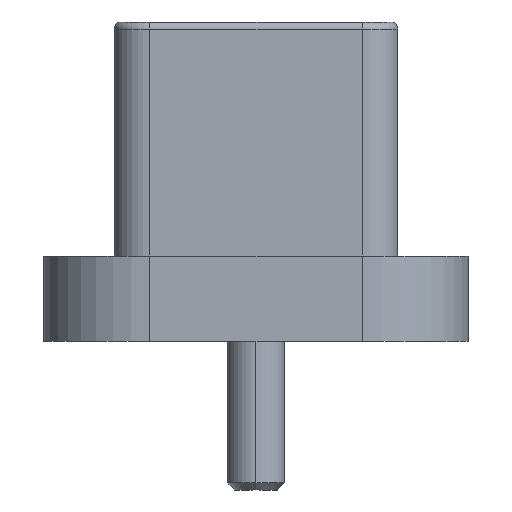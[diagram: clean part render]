
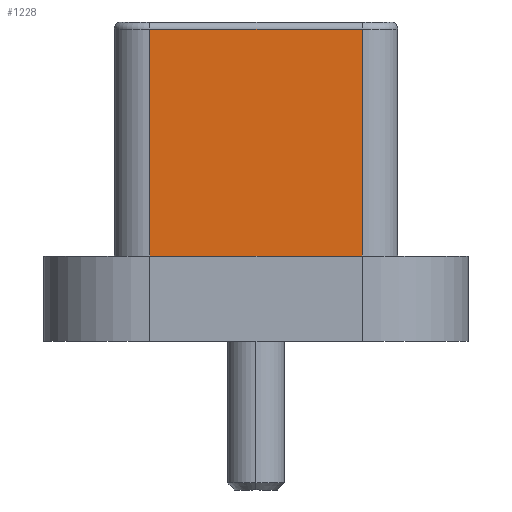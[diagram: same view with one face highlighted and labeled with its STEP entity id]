
A CAD part, left-side view. The second image highlights one B-rep face of the part: STEP entity #1228.
In plain terms, the highlighted planar face has unit normal (-1, 0, 0).
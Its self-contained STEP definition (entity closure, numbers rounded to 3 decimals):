
#111 = VERTEX_POINT ( 'NONE', #2740 ) ;
#316 = ORIENTED_EDGE ( 'NONE', *, *, #3835, .T. ) ;
#474 = CARTESIAN_POINT ( 'NONE',  ( -8.45, 1.5, -3.3 ) ) ;
#650 = LINE ( 'NONE', #2768, #5397 ) ;
#931 = VERTEX_POINT ( 'NONE', #3475 ) ;
#1100 = DIRECTION ( 'NONE',  ( 1., 0., 0. ) ) ;
#1228 = ADVANCED_FACE ( 'NONE', ( #1626 ), #3714, .F. ) ;
#1626 = FACE_OUTER_BOUND ( 'NONE', #5519, .T. ) ;
#1739 = VECTOR ( 'NONE', #6826, 1000. ) ;
#2544 = LINE ( 'NONE', #4677, #6033 ) ;
#2601 = DIRECTION ( 'NONE',  ( 0., -1., 0. ) ) ;
#2622 = LINE ( 'NONE', #4744, #1739 ) ;
#2649 = ORIENTED_EDGE ( 'NONE', *, *, #3925, .T. ) ;
#2740 = CARTESIAN_POINT ( 'NONE',  ( -8.45, 1.5, -3.3 ) ) ;
#2768 = CARTESIAN_POINT ( 'NONE',  ( -8.45, -1.5, -3.3 ) ) ;
#3069 = EDGE_CURVE ( 'NONE', #6422, #4673, #2622, .T. ) ;
#3185 = DIRECTION ( 'NONE',  ( 0., 1., 0. ) ) ;
#3358 = EDGE_CURVE ( 'NONE', #4673, #111, #2544, .T. ) ;
#3475 = CARTESIAN_POINT ( 'NONE',  ( -8.45, -1.5, -3.3 ) ) ;
#3714 = PLANE ( 'NONE',  #6267 ) ;
#3729 = CARTESIAN_POINT ( 'NONE',  ( -8.45, 1.5, -0.1 ) ) ;
#3835 = EDGE_CURVE ( 'NONE', #111, #931, #5246, .T. ) ;
#3925 = EDGE_CURVE ( 'NONE', #931, #6422, #650, .T. ) ;
#3983 = ORIENTED_EDGE ( 'NONE', *, *, #3069, .T. ) ;
#4673 = VERTEX_POINT ( 'NONE', #3729 ) ;
#4677 = CARTESIAN_POINT ( 'NONE',  ( -8.45, 1.5, -0.1 ) ) ;
#4744 = CARTESIAN_POINT ( 'NONE',  ( -8.45, -1.5, -0.1 ) ) ;
#4894 = DIRECTION ( 'NONE',  ( 0., 0., 1. ) ) ;
#5237 = CARTESIAN_POINT ( 'NONE',  ( -8.45, -1.5, -0.1 ) ) ;
#5246 = LINE ( 'NONE', #474, #6058 ) ;
#5397 = VECTOR ( 'NONE', #4894, 1000. ) ;
#5519 = EDGE_LOOP ( 'NONE', ( #6050, #316, #2649, #3983 ) ) ;
#5844 = CARTESIAN_POINT ( 'NONE',  ( -8.45, 0., -1.7 ) ) ;
#6033 = VECTOR ( 'NONE', #6759, 1000. ) ;
#6050 = ORIENTED_EDGE ( 'NONE', *, *, #3358, .T. ) ;
#6058 = VECTOR ( 'NONE', #2601, 1000. ) ;
#6267 = AXIS2_PLACEMENT_3D ( 'NONE', #5844, #1100, #3185 ) ;
#6422 = VERTEX_POINT ( 'NONE', #5237 ) ;
#6759 = DIRECTION ( 'NONE',  ( 0., 0., -1. ) ) ;
#6826 = DIRECTION ( 'NONE',  ( 0., 1., 0. ) ) ;
